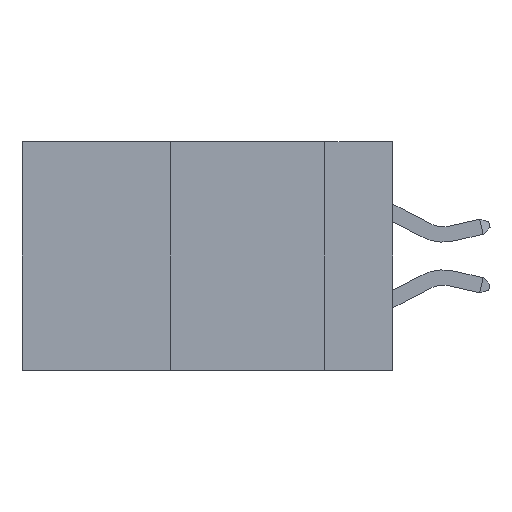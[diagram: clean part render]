
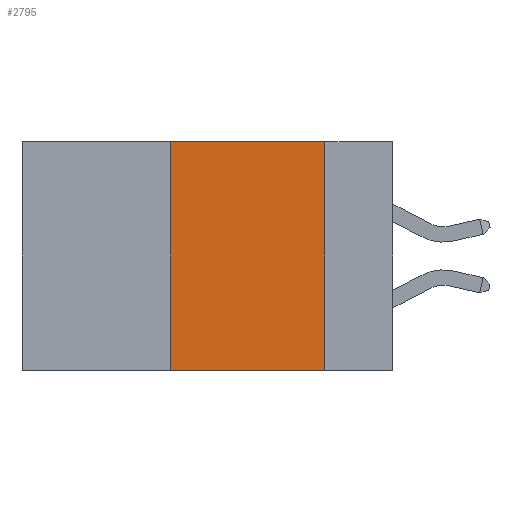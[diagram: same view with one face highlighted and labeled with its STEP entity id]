
A CAD part, left-side view. The second image highlights one B-rep face of the part: STEP entity #2795.
In plain terms, the highlighted planar face has unit normal (-1, 0, 0).
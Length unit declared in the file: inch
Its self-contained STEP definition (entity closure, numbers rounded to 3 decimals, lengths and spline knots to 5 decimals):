
#110 = LINE ( 'NONE', #7988, #10133 ) ;
#132 = DIRECTION ( 'NONE',  ( 0., -1., 0. ) ) ;
#726 = VERTEX_POINT ( 'NONE', #9758 ) ;
#840 = DIRECTION ( 'NONE',  ( 1., 0., 0. ) ) ;
#1240 = EDGE_CURVE ( 'NONE', #5063, #2574, #5529, .T. ) ;
#1298 = EDGE_LOOP ( 'NONE', ( #9676, #1954, #2537, #7530 ) ) ;
#1541 = CARTESIAN_POINT ( 'NONE',  ( 0., 0.6, 0. ) ) ;
#1954 = ORIENTED_EDGE ( 'NONE', *, *, #1240, .F. ) ;
#2133 = CARTESIAN_POINT ( 'NONE',  ( 0., 0.6, -0.37 ) ) ;
#2537 = ORIENTED_EDGE ( 'NONE', *, *, #9518, .F. ) ;
#2574 = VERTEX_POINT ( 'NONE', #4238 ) ;
#2795 = ADVANCED_FACE ( 'NONE', ( #5140 ), #10521, .F. ) ;
#3687 = CARTESIAN_POINT ( 'NONE',  ( 0., 0.6, 0. ) ) ;
#4238 = CARTESIAN_POINT ( 'NONE',  ( 0., 0.11, 0. ) ) ;
#4599 = EDGE_CURVE ( 'NONE', #5870, #726, #10912, .T. ) ;
#4892 = LINE ( 'NONE', #7929, #9666 ) ;
#5063 = VERTEX_POINT ( 'NONE', #10495 ) ;
#5140 = FACE_OUTER_BOUND ( 'NONE', #1298, .T. ) ;
#5529 = LINE ( 'NONE', #1541, #10008 ) ;
#5531 = AXIS2_PLACEMENT_3D ( 'NONE', #3687, #840, #8364 ) ;
#5870 = VERTEX_POINT ( 'NONE', #6957 ) ;
#6606 = EDGE_CURVE ( 'NONE', #2574, #726, #110, .T. ) ;
#6957 = CARTESIAN_POINT ( 'NONE',  ( 0., 0.36, -0.37 ) ) ;
#7530 = ORIENTED_EDGE ( 'NONE', *, *, #4599, .T. ) ;
#7929 = CARTESIAN_POINT ( 'NONE',  ( 0., 0.36, 0. ) ) ;
#7972 = DIRECTION ( 'NONE',  ( 0., 0., 1. ) ) ;
#7988 = CARTESIAN_POINT ( 'NONE',  ( 0., 0.11, 0. ) ) ;
#8032 = DIRECTION ( 'NONE',  ( 0., 0., -1. ) ) ;
#8364 = DIRECTION ( 'NONE',  ( 0., 0., -1. ) ) ;
#9036 = DIRECTION ( 'NONE',  ( 0., -1., 0. ) ) ;
#9518 = EDGE_CURVE ( 'NONE', #5870, #5063, #4892, .T. ) ;
#9666 = VECTOR ( 'NONE', #7972, 39.37008 ) ;
#9676 = ORIENTED_EDGE ( 'NONE', *, *, #6606, .F. ) ;
#9758 = CARTESIAN_POINT ( 'NONE',  ( 0., 0.11, -0.37 ) ) ;
#10008 = VECTOR ( 'NONE', #9036, 39.37008 ) ;
#10133 = VECTOR ( 'NONE', #8032, 39.37008 ) ;
#10495 = CARTESIAN_POINT ( 'NONE',  ( 0., 0.36, 0. ) ) ;
#10521 = PLANE ( 'NONE',  #5531 ) ;
#10625 = VECTOR ( 'NONE', #132, 39.37008 ) ;
#10912 = LINE ( 'NONE', #2133, #10625 ) ;
